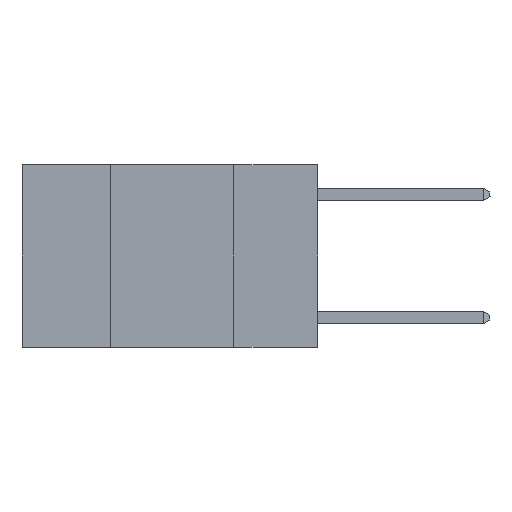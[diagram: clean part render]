
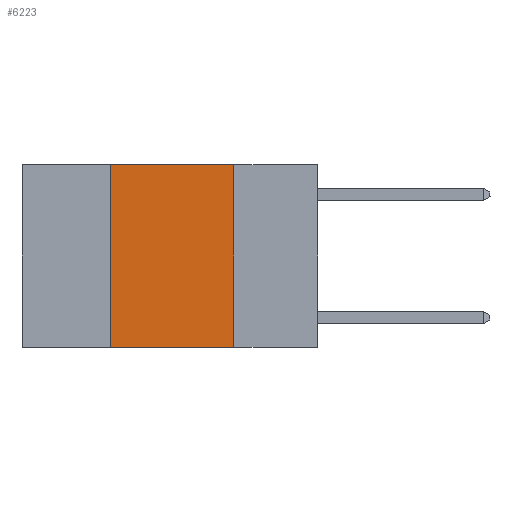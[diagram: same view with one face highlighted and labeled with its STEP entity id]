
A CAD part, left-side view. The second image highlights one B-rep face of the part: STEP entity #6223.
In plain terms, the highlighted planar face has unit normal (-1, 0, 0).
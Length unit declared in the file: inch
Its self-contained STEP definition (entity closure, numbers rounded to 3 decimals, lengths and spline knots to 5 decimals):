
#25 = ORIENTED_EDGE ( 'NONE', *, *, #471, .F. ) ;
#86 = ORIENTED_EDGE ( 'NONE', *, *, #7543, .F. ) ;
#233 = ORIENTED_EDGE ( 'NONE', *, *, #4896, .T. ) ;
#471 = EDGE_CURVE ( 'NONE', #2442, #8294, #9917, .T. ) ;
#1097 = EDGE_LOOP ( 'NONE', ( #5321, #25, #86, #233 ) ) ;
#1757 = CARTESIAN_POINT ( 'NONE',  ( 0., 0.17, -0.37 ) ) ;
#1837 = CARTESIAN_POINT ( 'NONE',  ( 0., 0.42, 0. ) ) ;
#1863 = CARTESIAN_POINT ( 'NONE',  ( 0., 0.6, 0. ) ) ;
#1969 = CARTESIAN_POINT ( 'NONE',  ( 0., 0.17, 0. ) ) ;
#2253 = VERTEX_POINT ( 'NONE', #2311 ) ;
#2311 = CARTESIAN_POINT ( 'NONE',  ( 0., 0.42, -0.37 ) ) ;
#2442 = VERTEX_POINT ( 'NONE', #5268 ) ;
#2623 = DIRECTION ( 'NONE',  ( 0., -1., 0. ) ) ;
#2857 = DIRECTION ( 'NONE',  ( 0., 0., -1. ) ) ;
#3601 = DIRECTION ( 'NONE',  ( 1., 0., 0. ) ) ;
#4251 = LINE ( 'NONE', #6892, #8676 ) ;
#4896 = EDGE_CURVE ( 'NONE', #2253, #10496, #4251, .T. ) ;
#5268 = CARTESIAN_POINT ( 'NONE',  ( 0., 0.42, 0. ) ) ;
#5321 = ORIENTED_EDGE ( 'NONE', *, *, #6982, .F. ) ;
#5936 = FACE_OUTER_BOUND ( 'NONE', #1097, .T. ) ;
#6223 = ADVANCED_FACE ( 'NONE', ( #5936 ), #8617, .F. ) ;
#6892 = CARTESIAN_POINT ( 'NONE',  ( 0., 0.6, -0.37 ) ) ;
#6982 = EDGE_CURVE ( 'NONE', #8294, #10496, #7870, .T. ) ;
#7543 = EDGE_CURVE ( 'NONE', #2253, #2442, #9474, .T. ) ;
#7618 = VECTOR ( 'NONE', #2857, 39.37008 ) ;
#7732 = AXIS2_PLACEMENT_3D ( 'NONE', #1863, #3601, #9421 ) ;
#7870 = LINE ( 'NONE', #1969, #7618 ) ;
#8294 = VERTEX_POINT ( 'NONE', #8521 ) ;
#8521 = CARTESIAN_POINT ( 'NONE',  ( 0., 0.17, 0. ) ) ;
#8617 = PLANE ( 'NONE',  #7732 ) ;
#8676 = VECTOR ( 'NONE', #2623, 39.37008 ) ;
#9234 = VECTOR ( 'NONE', #10193, 39.37008 ) ;
#9421 = DIRECTION ( 'NONE',  ( 0., 0., -1. ) ) ;
#9474 = LINE ( 'NONE', #1837, #9234 ) ;
#9651 = VECTOR ( 'NONE', #9929, 39.37008 ) ;
#9874 = CARTESIAN_POINT ( 'NONE',  ( 0., 0.6, 0. ) ) ;
#9917 = LINE ( 'NONE', #9874, #9651 ) ;
#9929 = DIRECTION ( 'NONE',  ( 0., -1., 0. ) ) ;
#10193 = DIRECTION ( 'NONE',  ( 0., 0., 1. ) ) ;
#10496 = VERTEX_POINT ( 'NONE', #1757 ) ;
